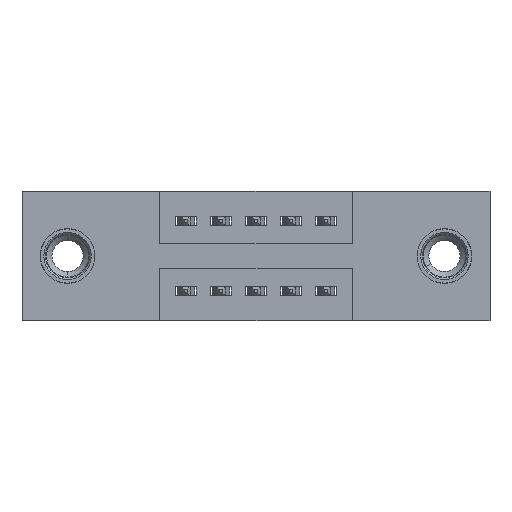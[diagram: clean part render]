
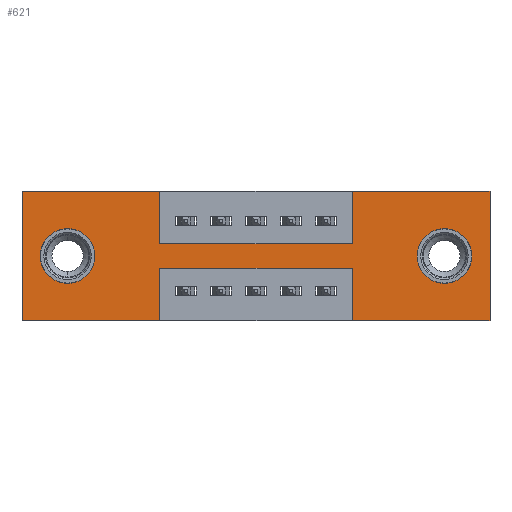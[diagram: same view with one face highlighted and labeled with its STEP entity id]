
A CAD part, front view. The second image highlights one B-rep face of the part: STEP entity #621.
In plain terms, the highlighted planar face has unit normal (0, -1, 0).
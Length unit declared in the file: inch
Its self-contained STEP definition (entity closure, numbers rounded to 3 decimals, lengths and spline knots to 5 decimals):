
#3 = CARTESIAN_POINT ( 'NONE',  ( 0., 0., -0.37 ) ) ;
#297 = CARTESIAN_POINT ( 'NONE',  ( 0.9425, 0., -0.15 ) ) ;
#325 = VERTEX_POINT ( 'NONE', #6854 ) ;
#416 = CARTESIAN_POINT ( 'NONE',  ( 1.335, 0., 0. ) ) ;
#612 = CARTESIAN_POINT ( 'NONE',  ( 0.13, 0., -0.185 ) ) ;
#621 = ADVANCED_FACE ( 'NONE', ( #2068, #4106, #1804 ), #3095, .T. ) ;
#724 = EDGE_CURVE ( 'NONE', #5348, #3689, #4223, .T. ) ;
#900 = EDGE_LOOP ( 'NONE', ( #8252, #6118, #2207, #5282, #4206, #2895, #5132, #4075, #2476, #7732, #9569, #3355 ) ) ;
#1044 = EDGE_CURVE ( 'NONE', #2969, #8670, #7315, .T. ) ;
#1219 = LINE ( 'NONE', #1338, #9129 ) ;
#1238 = VERTEX_POINT ( 'NONE', #5345 ) ;
#1257 = VERTEX_POINT ( 'NONE', #7632 ) ;
#1318 = CARTESIAN_POINT ( 'NONE',  ( 1.205, 0., -0.185 ) ) ;
#1338 = CARTESIAN_POINT ( 'NONE',  ( 0.3925, 0., 0. ) ) ;
#1457 = DIRECTION ( 'NONE',  ( 0., 0., -1. ) ) ;
#1486 = CARTESIAN_POINT ( 'NONE',  ( 0.9425, 0., 0. ) ) ;
#1591 = DIRECTION ( 'NONE',  ( 0., 0., 1. ) ) ;
#1688 = EDGE_CURVE ( 'NONE', #3031, #325, #3842, .T. ) ;
#1804 = FACE_OUTER_BOUND ( 'NONE', #900, .T. ) ;
#2067 = AXIS2_PLACEMENT_3D ( 'NONE', #2789, #8088, #3562 ) ;
#2068 = FACE_BOUND ( 'NONE', #9013, .T. ) ;
#2194 = DIRECTION ( 'NONE',  ( 0., 0., -1. ) ) ;
#2207 = ORIENTED_EDGE ( 'NONE', *, *, #9048, .F. ) ;
#2255 = VECTOR ( 'NONE', #3100, 39.37008 ) ;
#2476 = ORIENTED_EDGE ( 'NONE', *, *, #5439, .F. ) ;
#2488 = EDGE_LOOP ( 'NONE', ( #6757, #8431 ) ) ;
#2789 = CARTESIAN_POINT ( 'NONE',  ( 1.205, 0., -0.185 ) ) ;
#2878 = CIRCLE ( 'NONE', #4315, 0.078 ) ;
#2895 = ORIENTED_EDGE ( 'NONE', *, *, #7820, .F. ) ;
#2969 = VERTEX_POINT ( 'NONE', #7203 ) ;
#3031 = VERTEX_POINT ( 'NONE', #5763 ) ;
#3048 = AXIS2_PLACEMENT_3D ( 'NONE', #1318, #6761, #2194 ) ;
#3095 = PLANE ( 'NONE',  #8039 ) ;
#3100 = DIRECTION ( 'NONE',  ( 0., 0., 1. ) ) ;
#3172 = VECTOR ( 'NONE', #8877, 39.37008 ) ;
#3288 = EDGE_CURVE ( 'NONE', #1238, #6244, #8714, .T. ) ;
#3355 = ORIENTED_EDGE ( 'NONE', *, *, #4372, .F. ) ;
#3562 = DIRECTION ( 'NONE',  ( 0., 0., -1. ) ) ;
#3606 = VECTOR ( 'NONE', #6539, 39.37008 ) ;
#3608 = CARTESIAN_POINT ( 'NONE',  ( 0.3925, 0., 0. ) ) ;
#3689 = VERTEX_POINT ( 'NONE', #1486 ) ;
#3783 = VERTEX_POINT ( 'NONE', #4715 ) ;
#3802 = LINE ( 'NONE', #5393, #2255 ) ;
#3816 = VERTEX_POINT ( 'NONE', #7756 ) ;
#3842 = LINE ( 'NONE', #9350, #9781 ) ;
#3923 = ORIENTED_EDGE ( 'NONE', *, *, #3288, .T. ) ;
#4046 = DIRECTION ( 'NONE',  ( 0., -1., 0. ) ) ;
#4075 = ORIENTED_EDGE ( 'NONE', *, *, #9713, .F. ) ;
#4106 = FACE_BOUND ( 'NONE', #2488, .T. ) ;
#4118 = EDGE_CURVE ( 'NONE', #6131, #9211, #8593, .T. ) ;
#4206 = ORIENTED_EDGE ( 'NONE', *, *, #4118, .F. ) ;
#4223 = LINE ( 'NONE', #7218, #8242 ) ;
#4226 = DIRECTION ( 'NONE',  ( 0., 0., -1. ) ) ;
#4315 = AXIS2_PLACEMENT_3D ( 'NONE', #612, #6217, #1591 ) ;
#4321 = EDGE_CURVE ( 'NONE', #10087, #6729, #9145, .T. ) ;
#4372 = EDGE_CURVE ( 'NONE', #325, #3816, #4954, .T. ) ;
#4427 = CARTESIAN_POINT ( 'NONE',  ( 0.3925, 0., -0.15 ) ) ;
#4430 = CARTESIAN_POINT ( 'NONE',  ( 0., 0., -0.37 ) ) ;
#4545 = LINE ( 'NONE', #9509, #6324 ) ;
#4715 = CARTESIAN_POINT ( 'NONE',  ( 0.9425, 0., -0.22 ) ) ;
#4861 = DIRECTION ( 'NONE',  ( -1., 0., 0. ) ) ;
#4880 = EDGE_CURVE ( 'NONE', #3783, #3031, #8910, .T. ) ;
#4920 = CARTESIAN_POINT ( 'NONE',  ( 0.13, 0., -0.185 ) ) ;
#4954 = LINE ( 'NONE', #4430, #8699 ) ;
#4966 = CARTESIAN_POINT ( 'NONE',  ( 1.335, 0., 0. ) ) ;
#5132 = ORIENTED_EDGE ( 'NONE', *, *, #724, .F. ) ;
#5155 = CIRCLE ( 'NONE', #2067, 0.078 ) ;
#5282 = ORIENTED_EDGE ( 'NONE', *, *, #8708, .F. ) ;
#5345 = CARTESIAN_POINT ( 'NONE',  ( 1.205, 0., -0.107 ) ) ;
#5348 = VERTEX_POINT ( 'NONE', #297 ) ;
#5354 = ORIENTED_EDGE ( 'NONE', *, *, #7873, .T. ) ;
#5375 = CARTESIAN_POINT ( 'NONE',  ( 0.9425, 0., -0.37 ) ) ;
#5393 = CARTESIAN_POINT ( 'NONE',  ( 0., 0., 0. ) ) ;
#5439 = EDGE_CURVE ( 'NONE', #6729, #1257, #1219, .T. ) ;
#5496 = DIRECTION ( 'NONE',  ( 0., 0., 1. ) ) ;
#5629 = LINE ( 'NONE', #5777, #3606 ) ;
#5657 = DIRECTION ( 'NONE',  ( 0., 0., -1. ) ) ;
#5677 = DIRECTION ( 'NONE',  ( 0., 0., 1. ) ) ;
#5763 = CARTESIAN_POINT ( 'NONE',  ( 0.3925, 0., -0.22 ) ) ;
#5777 = CARTESIAN_POINT ( 'NONE',  ( 0., 0., 0. ) ) ;
#5838 = DIRECTION ( 'NONE',  ( -1., 0., 0. ) ) ;
#5958 = LINE ( 'NONE', #5375, #9643 ) ;
#6118 = ORIENTED_EDGE ( 'NONE', *, *, #4880, .F. ) ;
#6129 = DIRECTION ( 'NONE',  ( 0., 0., 1. ) ) ;
#6131 = VERTEX_POINT ( 'NONE', #416 ) ;
#6212 = DIRECTION ( 'NONE',  ( 0., 0., -1. ) ) ;
#6217 = DIRECTION ( 'NONE',  ( 0., 1., 0. ) ) ;
#6244 = VERTEX_POINT ( 'NONE', #8430 ) ;
#6324 = VECTOR ( 'NONE', #5838, 39.37008 ) ;
#6352 = CARTESIAN_POINT ( 'NONE',  ( 0.3925, 0., -0.22 ) ) ;
#6539 = DIRECTION ( 'NONE',  ( 1., 0., 0. ) ) ;
#6611 = VECTOR ( 'NONE', #4226, 39.37008 ) ;
#6653 = CARTESIAN_POINT ( 'NONE',  ( 0., 0., 0. ) ) ;
#6729 = VERTEX_POINT ( 'NONE', #3608 ) ;
#6757 = ORIENTED_EDGE ( 'NONE', *, *, #1044, .T. ) ;
#6761 = DIRECTION ( 'NONE',  ( 0., 1., 0. ) ) ;
#6783 = VECTOR ( 'NONE', #7489, 39.37008 ) ;
#6788 = CARTESIAN_POINT ( 'NONE',  ( 0.9425, 0., -0.37 ) ) ;
#6854 = CARTESIAN_POINT ( 'NONE',  ( 0.3925, 0., -0.37 ) ) ;
#6965 = VECTOR ( 'NONE', #4861, 39.37008 ) ;
#7048 = CARTESIAN_POINT ( 'NONE',  ( 0., 0., 0. ) ) ;
#7115 = EDGE_CURVE ( 'NONE', #8670, #2969, #2878, .T. ) ;
#7203 = CARTESIAN_POINT ( 'NONE',  ( 0.13, 0., -0.107 ) ) ;
#7218 = CARTESIAN_POINT ( 'NONE',  ( 0.9425, 0., 0. ) ) ;
#7315 = CIRCLE ( 'NONE', #9349, 0.078 ) ;
#7489 = DIRECTION ( 'NONE',  ( 1., 0., 0. ) ) ;
#7632 = CARTESIAN_POINT ( 'NONE',  ( 0.3925, 0., -0.15 ) ) ;
#7732 = ORIENTED_EDGE ( 'NONE', *, *, #4321, .F. ) ;
#7756 = CARTESIAN_POINT ( 'NONE',  ( 0., 0., -0.37 ) ) ;
#7820 = EDGE_CURVE ( 'NONE', #3689, #6131, #5629, .T. ) ;
#7873 = EDGE_CURVE ( 'NONE', #6244, #1238, #5155, .T. ) ;
#8039 = AXIS2_PLACEMENT_3D ( 'NONE', #3, #4046, #6212 ) ;
#8047 = CARTESIAN_POINT ( 'NONE',  ( 0.13, 0., -0.263 ) ) ;
#8088 = DIRECTION ( 'NONE',  ( 0., 1., 0. ) ) ;
#8242 = VECTOR ( 'NONE', #5496, 39.37008 ) ;
#8252 = ORIENTED_EDGE ( 'NONE', *, *, #1688, .F. ) ;
#8430 = CARTESIAN_POINT ( 'NONE',  ( 1.205, 0., -0.263 ) ) ;
#8431 = ORIENTED_EDGE ( 'NONE', *, *, #7115, .T. ) ;
#8593 = LINE ( 'NONE', #4966, #6611 ) ;
#8670 = VERTEX_POINT ( 'NONE', #8047 ) ;
#8699 = VECTOR ( 'NONE', #9629, 39.37008 ) ;
#8708 = EDGE_CURVE ( 'NONE', #9211, #9802, #4545, .T. ) ;
#8714 = CIRCLE ( 'NONE', #3048, 0.078 ) ;
#8737 = LINE ( 'NONE', #4427, #6783 ) ;
#8877 = DIRECTION ( 'NONE',  ( 1., 0., 0. ) ) ;
#8910 = LINE ( 'NONE', #6352, #6965 ) ;
#9013 = EDGE_LOOP ( 'NONE', ( #3923, #5354 ) ) ;
#9048 = EDGE_CURVE ( 'NONE', #9802, #3783, #5958, .T. ) ;
#9129 = VECTOR ( 'NONE', #1457, 39.37008 ) ;
#9145 = LINE ( 'NONE', #6653, #3172 ) ;
#9197 = CARTESIAN_POINT ( 'NONE',  ( 1.335, 0., -0.37 ) ) ;
#9211 = VERTEX_POINT ( 'NONE', #9197 ) ;
#9349 = AXIS2_PLACEMENT_3D ( 'NONE', #4920, #10076, #5677 ) ;
#9350 = CARTESIAN_POINT ( 'NONE',  ( 0.3925, 0., -0.37 ) ) ;
#9509 = CARTESIAN_POINT ( 'NONE',  ( 0., 0., -0.37 ) ) ;
#9569 = ORIENTED_EDGE ( 'NONE', *, *, #9914, .F. ) ;
#9629 = DIRECTION ( 'NONE',  ( -1., 0., 0. ) ) ;
#9643 = VECTOR ( 'NONE', #6129, 39.37008 ) ;
#9713 = EDGE_CURVE ( 'NONE', #1257, #5348, #8737, .T. ) ;
#9781 = VECTOR ( 'NONE', #5657, 39.37008 ) ;
#9802 = VERTEX_POINT ( 'NONE', #6788 ) ;
#9914 = EDGE_CURVE ( 'NONE', #3816, #10087, #3802, .T. ) ;
#10076 = DIRECTION ( 'NONE',  ( 0., 1., 0. ) ) ;
#10087 = VERTEX_POINT ( 'NONE', #7048 ) ;
